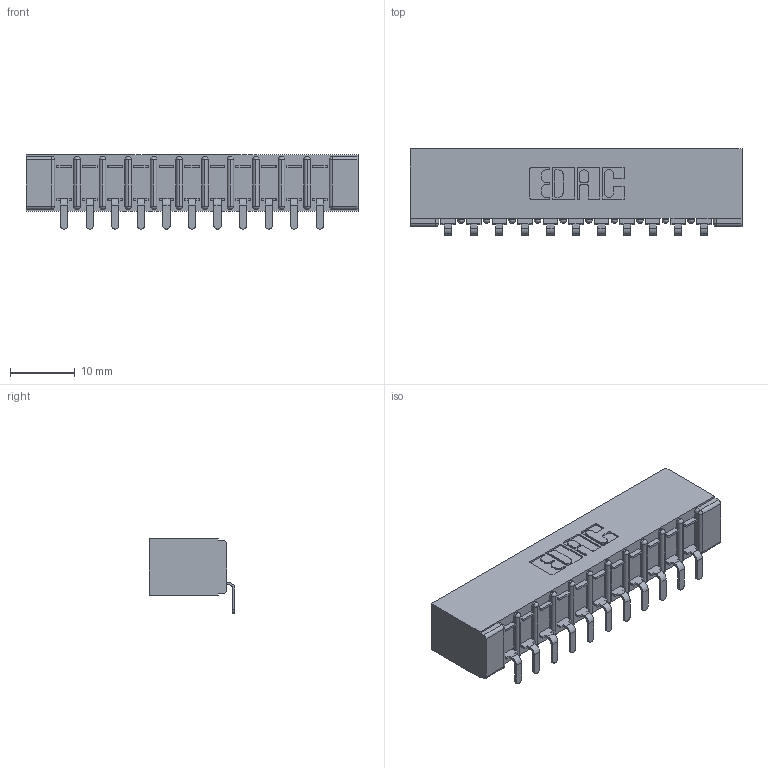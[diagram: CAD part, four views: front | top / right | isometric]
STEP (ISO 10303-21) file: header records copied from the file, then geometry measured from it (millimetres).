
FILE_DESCRIPTION (( 'STEP AP203' ), '1' );
FILE_NAME ('357-011-553-101.STEP', '2019-09-16T18:53:44', ( '' ), ( '' ), 'SwSTEP 2.0', 'SolidWorks 2016', '' );
FILE_SCHEMA (( 'CONFIG_CONTROL_DESIGN' ));
Length unit declared in the file: inch
Products named in the file (3): 357-011-553-101; 307-290-002_553; 307 Part_No Mounting Lugs
Assembly tree (12 placements, depth 2):
  357-011-553-101
    307 Part_No Mounting Lugs
    307-290-002_553  x11
Bounding box: 51.46 x 13.32 x 11.51 mm (x, y, z)
Volume: 3633.8 mm3; surface area: 6508.2 mm2
Topology: 12 solids, 12 shells, 980 faces, 2983 edges, 1954 vertices
Faces by surface type: plane 583, cylinder 373, sphere 24
Entity records: 13828 total; most frequent: CARTESIAN_POINT 2328, ORIENTED_EDGE 2318, DIRECTION 2275, EDGE_CURVE 1159, LINE 873, VECTOR 873, VERTEX_POINT 754, AXIS2_PLACEMENT_3D 701
